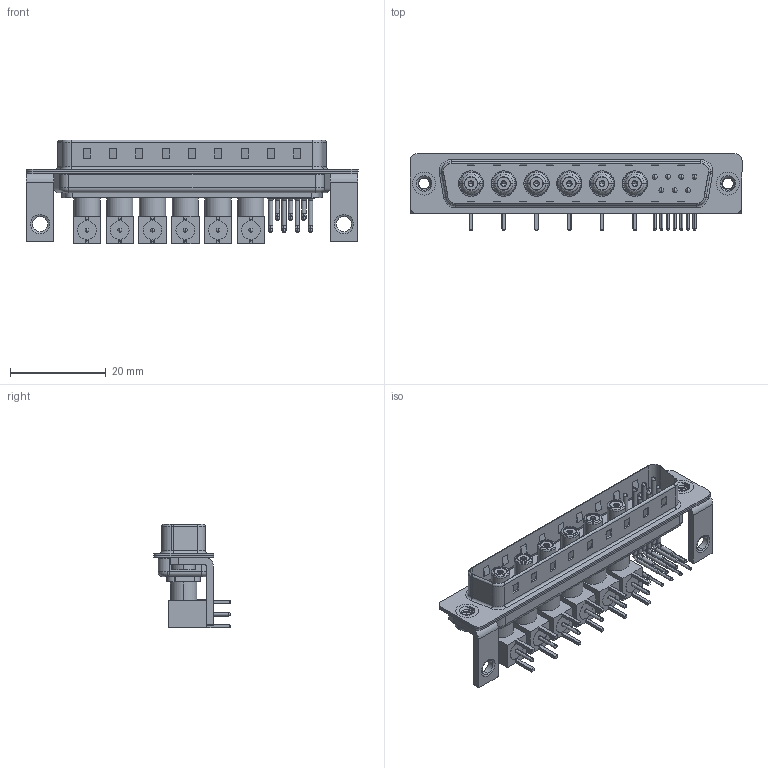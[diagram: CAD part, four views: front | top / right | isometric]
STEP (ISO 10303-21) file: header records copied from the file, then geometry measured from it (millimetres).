
FILE_DESCRIPTION (( 'STEP AP203' ), '1' );
FILE_NAME ('629-13W6640-5TC.STEP', '2022-05-14T19:01:03', ( '' ), ( '' ), 'SwSTEP 2.0', 'SolidWorks 2020', '' );
FILE_SCHEMA (( 'CONFIG_CONTROL_DESIGN' ));
Length unit declared in the file: millimetre
Products named in the file (21): Co-Ax Jack Assy_RA; 629-13W6640-5TC; 629Combo Contact Row 1; Socket_RA; Insulator Socket; 629Combo Shell Front_37 Contacts; Insulator Socket 2; 629Combo Housing_13W6; RA Back Shell; 629Combo Contact Row 2; 629Combo Stabilizer Bracket; Co-Ax Jack_RA PC Tail; 629Combo Shell Rear_37 Contacts; Insulator RA Pin; Locking Collar; 629Combo Threaded Rivet_2
Assembly tree (62 placements, depth 3):
  629-13W6640-5TC
    629Combo Housing_13W6
    629Combo Shell Rear_37 Contacts
    629Combo Shell Front_37 Contacts
    629Combo Threaded Rivet_2  x2
    629Combo Stabilizer Bracket  x2
    Co-Ax Jack Assy_RA
      Co-Ax Jack_RA PC Tail
      Insulator Socket
      Insulator Socket 2
      Locking Collar
      Socket_RA
      RA Back Shell
      Insulator RA Pin
    Co-Ax Jack Assy_RA
      Co-Ax Jack_RA PC Tail
      Insulator Socket
      Insulator Socket 2
      Locking Collar
      Socket_RA
      RA Back Shell
      Insulator RA Pin
    Co-Ax Jack Assy_RA
      Co-Ax Jack_RA PC Tail
      Insulator Socket
      Insulator Socket 2
      Locking Collar
      Socket_RA
      RA Back Shell
      Insulator RA Pin
    Co-Ax Jack Assy_RA
      Co-Ax Jack_RA PC Tail
      Insulator Socket
      Insulator Socket 2
      Locking Collar
      Socket_RA
      RA Back Shell
      Insulator RA Pin
    Co-Ax Jack Assy_RA
      Co-Ax Jack_RA PC Tail
      Insulator Socket
      Insulator Socket 2
      Locking Collar
      Socket_RA
      RA Back Shell
      Insulator RA Pin
    Co-Ax Jack Assy_RA
      Co-Ax Jack_RA PC Tail
      Insulator Socket
      Insulator Socket 2
      Locking Collar
      Socket_RA
      RA Back Shell
      Insulator RA Pin
    629Combo Contact Row 1  x4
    629Combo Contact Row 2  x3
Bounding box: 69.4 x 16 x 21.71 mm (x, y, z)
Volume: 5849 mm3; surface area: 15593.1 mm2
Topology: 56 solids, 56 shells, 2142 faces, 5433 edges, 3450 vertices
Faces by surface type: plane 1013, cylinder 819, cone 158, torus 86, bspline 54, sphere 12
Entity records: 30850 total; most frequent: CARTESIAN_POINT 6331, DIRECTION 4620, ORIENTED_EDGE 4274, EDGE_CURVE 2137, AXIS2_PLACEMENT_3D 1653, VERTEX_POINT 1373, VECTOR 1314, LINE 1314
